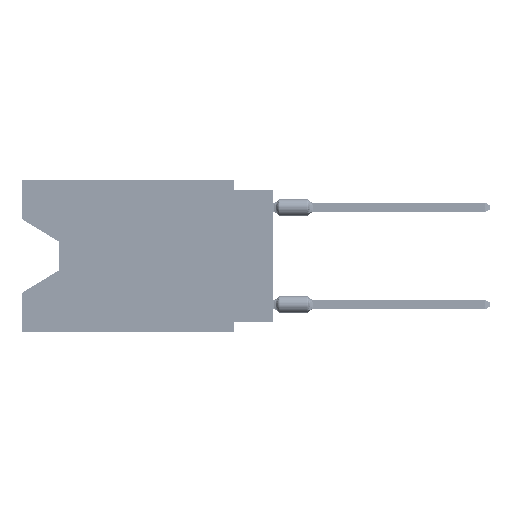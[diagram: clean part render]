
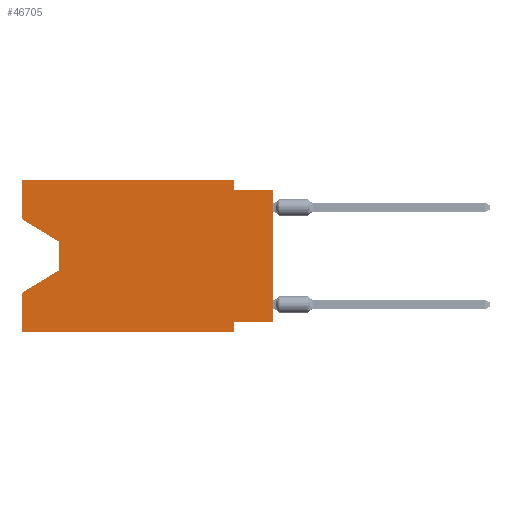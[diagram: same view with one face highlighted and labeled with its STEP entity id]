
A CAD part, left-side view. The second image highlights one B-rep face of the part: STEP entity #46705.
In plain terms, the highlighted planar face has unit normal (-1, 0, 0).
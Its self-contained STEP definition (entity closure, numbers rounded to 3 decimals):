
#68 = VERTEX_POINT ( 'NONE', #1014 ) ;
#182 = EDGE_CURVE ( 'NONE', #57137, #38327, #65835, .T. ) ;
#209 = VERTEX_POINT ( 'NONE', #53003 ) ;
#339 = VECTOR ( 'NONE', #62250, 1000. ) ;
#911 = VERTEX_POINT ( 'NONE', #32755 ) ;
#1014 = CARTESIAN_POINT ( 'NONE',  ( 0., 16.383, -7.36 ) ) ;
#1724 = CARTESIAN_POINT ( 'NONE',  ( 0., 0., -9.271 ) ) ;
#1725 = CARTESIAN_POINT ( 'NONE',  ( 0., 2.54, 0. ) ) ;
#2053 = ORIENTED_EDGE ( 'NONE', *, *, #182, .F. ) ;
#2149 = VECTOR ( 'NONE', #19901, 1000. ) ;
#3455 = VECTOR ( 'NONE', #19468, 1000. ) ;
#3581 = EDGE_CURVE ( 'NONE', #40880, #11794, #58316, .T. ) ;
#4735 = ORIENTED_EDGE ( 'NONE', *, *, #5311, .F. ) ;
#5026 = ORIENTED_EDGE ( 'NONE', *, *, #34487, .F. ) ;
#5311 = EDGE_CURVE ( 'NONE', #209, #57137, #65289, .T. ) ;
#6035 = ORIENTED_EDGE ( 'NONE', *, *, #52120, .T. ) ;
#6180 = CARTESIAN_POINT ( 'NONE',  ( 0., 13.97, -4.013 ) ) ;
#6685 = CARTESIAN_POINT ( 'NONE',  ( 0., 16.383, -2.546 ) ) ;
#7364 = DIRECTION ( 'NONE',  ( 0., 0.855, -0.519 ) ) ;
#7775 = LINE ( 'NONE', #57761, #22821 ) ;
#11794 = VERTEX_POINT ( 'NONE', #70988 ) ;
#14003 = VERTEX_POINT ( 'NONE', #69572 ) ;
#14704 = ORIENTED_EDGE ( 'NONE', *, *, #49325, .T. ) ;
#14821 = DIRECTION ( 'NONE',  ( 0., 0., -1. ) ) ;
#15683 = CARTESIAN_POINT ( 'NONE',  ( 0., 0., -9.271 ) ) ;
#17862 = EDGE_CURVE ( 'NONE', #38327, #14003, #77558, .T. ) ;
#19119 = FACE_OUTER_BOUND ( 'NONE', #22953, .T. ) ;
#19468 = DIRECTION ( 'NONE',  ( 0., -1., 0. ) ) ;
#19901 = DIRECTION ( 'NONE',  ( 0., 1., 0. ) ) ;
#20332 = DIRECTION ( 'NONE',  ( 1., 0., 0. ) ) ;
#21335 = VECTOR ( 'NONE', #72761, 1000. ) ;
#21775 = CARTESIAN_POINT ( 'NONE',  ( 0., 0., -0.635 ) ) ;
#21913 = VECTOR ( 'NONE', #65148, 1000. ) ;
#22411 = LINE ( 'NONE', #47590, #21335 ) ;
#22821 = VECTOR ( 'NONE', #7364, 1000. ) ;
#22953 = EDGE_LOOP ( 'NONE', ( #14704, #50312, #73549, #51747, #6035, #55982, #39868, #41149, #37757, #2053, #4735, #5026 ) ) ;
#23283 = VERTEX_POINT ( 'NONE', #6685 ) ;
#27643 = DIRECTION ( 'NONE',  ( 0., 0., 1. ) ) ;
#28332 = LINE ( 'NONE', #67542, #73948 ) ;
#30479 = LINE ( 'NONE', #68451, #339 ) ;
#32748 = CARTESIAN_POINT ( 'NONE',  ( 0., 16.383, 0. ) ) ;
#32755 = CARTESIAN_POINT ( 'NONE',  ( 0., 16.383, -9.906 ) ) ;
#33494 = CARTESIAN_POINT ( 'NONE',  ( 0., 16.383, 0. ) ) ;
#33806 = CARTESIAN_POINT ( 'NONE',  ( 0., 2.54, -9.906 ) ) ;
#34032 = CARTESIAN_POINT ( 'NONE',  ( 0., 13.97, -4.013 ) ) ;
#34487 = EDGE_CURVE ( 'NONE', #23283, #209, #28332, .T. ) ;
#34618 = LINE ( 'NONE', #53609, #70394 ) ;
#35841 = VECTOR ( 'NONE', #59226, 1000. ) ;
#36070 = DIRECTION ( 'NONE',  ( 0., 0., -1. ) ) ;
#36753 = EDGE_CURVE ( 'NONE', #51114, #68, #7775, .T. ) ;
#37757 = ORIENTED_EDGE ( 'NONE', *, *, #17862, .F. ) ;
#38072 = EDGE_CURVE ( 'NONE', #911, #68, #34618, .T. ) ;
#38327 = VERTEX_POINT ( 'NONE', #57671 ) ;
#39856 = VERTEX_POINT ( 'NONE', #57597 ) ;
#39868 = ORIENTED_EDGE ( 'NONE', *, *, #3581, .F. ) ;
#40880 = VERTEX_POINT ( 'NONE', #15683 ) ;
#41149 = ORIENTED_EDGE ( 'NONE', *, *, #53007, .T. ) ;
#42244 = VECTOR ( 'NONE', #14821, 1000. ) ;
#42611 = VECTOR ( 'NONE', #36070, 1000. ) ;
#45525 = DIRECTION ( 'NONE',  ( 0., 0., -1. ) ) ;
#46192 = DIRECTION ( 'NONE',  ( 0., 0., 1. ) ) ;
#46705 = ADVANCED_FACE ( 'NONE', ( #19119 ), #76929, .F. ) ;
#47590 = CARTESIAN_POINT ( 'NONE',  ( 0., 16.383, -2.546 ) ) ;
#49325 = EDGE_CURVE ( 'NONE', #23283, #60715, #22411, .T. ) ;
#50312 = ORIENTED_EDGE ( 'NONE', *, *, #52696, .T. ) ;
#50706 = EDGE_CURVE ( 'NONE', #11794, #39856, #71373, .T. ) ;
#51114 = VERTEX_POINT ( 'NONE', #58902 ) ;
#51747 = ORIENTED_EDGE ( 'NONE', *, *, #38072, .F. ) ;
#52120 = EDGE_CURVE ( 'NONE', #911, #39856, #30479, .T. ) ;
#52696 = EDGE_CURVE ( 'NONE', #60715, #51114, #70368, .T. ) ;
#53003 = CARTESIAN_POINT ( 'NONE',  ( 0., 16.383, 0. ) ) ;
#53007 = EDGE_CURVE ( 'NONE', #40880, #14003, #59027, .T. ) ;
#53609 = CARTESIAN_POINT ( 'NONE',  ( 0., 16.383, 0. ) ) ;
#55329 = AXIS2_PLACEMENT_3D ( 'NONE', #32748, #20332, #45525 ) ;
#55982 = ORIENTED_EDGE ( 'NONE', *, *, #50706, .F. ) ;
#57137 = VERTEX_POINT ( 'NONE', #1725 ) ;
#57597 = CARTESIAN_POINT ( 'NONE',  ( 0., 2.54, -9.906 ) ) ;
#57671 = CARTESIAN_POINT ( 'NONE',  ( 0., 2.54, -0.635 ) ) ;
#57761 = CARTESIAN_POINT ( 'NONE',  ( 0., 13.97, -5.893 ) ) ;
#58316 = LINE ( 'NONE', #1724, #2149 ) ;
#58902 = CARTESIAN_POINT ( 'NONE',  ( 0., 13.97, -5.893 ) ) ;
#59027 = LINE ( 'NONE', #70995, #64832 ) ;
#59226 = DIRECTION ( 'NONE',  ( 0., 0., -1. ) ) ;
#60715 = VERTEX_POINT ( 'NONE', #6180 ) ;
#62250 = DIRECTION ( 'NONE',  ( 0., -1., 0. ) ) ;
#64832 = VECTOR ( 'NONE', #27643, 1000. ) ;
#65148 = DIRECTION ( 'NONE',  ( 0., -1., 0. ) ) ;
#65289 = LINE ( 'NONE', #33494, #3455 ) ;
#65835 = LINE ( 'NONE', #78219, #42611 ) ;
#67542 = CARTESIAN_POINT ( 'NONE',  ( 0., 16.383, 0. ) ) ;
#68451 = CARTESIAN_POINT ( 'NONE',  ( 0., 16.383, -9.906 ) ) ;
#69572 = CARTESIAN_POINT ( 'NONE',  ( 0., 0., -0.635 ) ) ;
#70368 = LINE ( 'NONE', #34032, #35841 ) ;
#70394 = VECTOR ( 'NONE', #46192, 1000. ) ;
#70988 = CARTESIAN_POINT ( 'NONE',  ( 0., 2.54, -9.271 ) ) ;
#70995 = CARTESIAN_POINT ( 'NONE',  ( 0., 0., 0. ) ) ;
#71373 = LINE ( 'NONE', #33806, #42244 ) ;
#72761 = DIRECTION ( 'NONE',  ( 0., -0.855, -0.519 ) ) ;
#73324 = DIRECTION ( 'NONE',  ( 0., 0., 1. ) ) ;
#73549 = ORIENTED_EDGE ( 'NONE', *, *, #36753, .T. ) ;
#73948 = VECTOR ( 'NONE', #73324, 1000. ) ;
#76929 = PLANE ( 'NONE',  #55329 ) ;
#77558 = LINE ( 'NONE', #21775, #21913 ) ;
#78219 = CARTESIAN_POINT ( 'NONE',  ( 0., 2.54, 0. ) ) ;
